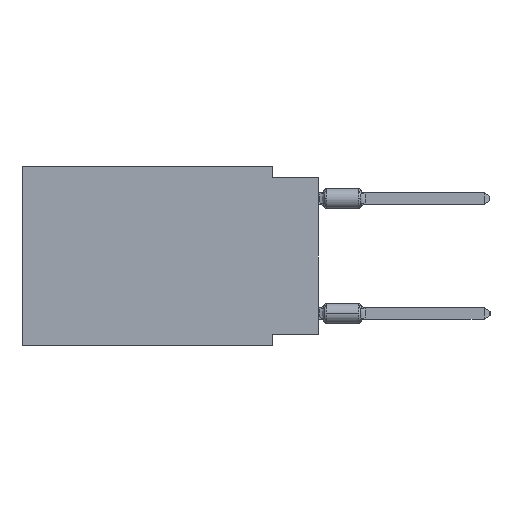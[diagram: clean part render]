
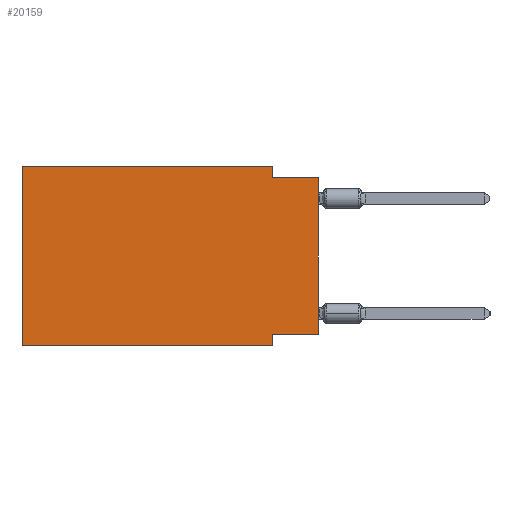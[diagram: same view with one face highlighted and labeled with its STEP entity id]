
A CAD part, left-side view. The second image highlights one B-rep face of the part: STEP entity #20159.
In plain terms, the highlighted planar face has unit normal (-1, 0, 0).
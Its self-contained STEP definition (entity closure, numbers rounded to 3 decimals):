
#829 = DIRECTION ( 'NONE',  ( 0., 0., -1. ) ) ;
#1576 = VERTEX_POINT ( 'NONE', #36113 ) ;
#1631 = ORIENTED_EDGE ( 'NONE', *, *, #31599, .T. ) ;
#2872 = VECTOR ( 'NONE', #36932, 1000. ) ;
#3342 = CARTESIAN_POINT ( 'NONE',  ( 0., 16.383, 0. ) ) ;
#4728 = CARTESIAN_POINT ( 'NONE',  ( 0., 0., -9.271 ) ) ;
#4975 = PLANE ( 'NONE',  #40222 ) ;
#6924 = VERTEX_POINT ( 'NONE', #50520 ) ;
#7307 = VERTEX_POINT ( 'NONE', #45856 ) ;
#8374 = VERTEX_POINT ( 'NONE', #40048 ) ;
#9286 = EDGE_LOOP ( 'NONE', ( #39511, #28582, #34691, #48635, #46377, #1631, #33042, #9824 ) ) ;
#9824 = ORIENTED_EDGE ( 'NONE', *, *, #44631, .F. ) ;
#10026 = CARTESIAN_POINT ( 'NONE',  ( 0., 16.383, 0. ) ) ;
#10186 = DIRECTION ( 'NONE',  ( 0., 0., -1. ) ) ;
#11229 = LINE ( 'NONE', #38233, #13995 ) ;
#12120 = VERTEX_POINT ( 'NONE', #58046 ) ;
#13102 = EDGE_CURVE ( 'NONE', #1576, #8374, #18227, .T. ) ;
#13995 = VECTOR ( 'NONE', #829, 1000. ) ;
#16010 = VECTOR ( 'NONE', #32621, 1000. ) ;
#18227 = LINE ( 'NONE', #41234, #2872 ) ;
#18235 = LINE ( 'NONE', #4728, #16010 ) ;
#19677 = FACE_OUTER_BOUND ( 'NONE', #9286, .T. ) ;
#19977 = EDGE_CURVE ( 'NONE', #7307, #20957, #27353, .T. ) ;
#20159 = ADVANCED_FACE ( 'NONE', ( #19677 ), #4975, .F. ) ;
#20957 = VERTEX_POINT ( 'NONE', #35305 ) ;
#23691 = VERTEX_POINT ( 'NONE', #58237 ) ;
#27317 = EDGE_CURVE ( 'NONE', #6924, #37958, #49645, .T. ) ;
#27353 = LINE ( 'NONE', #31956, #49989 ) ;
#28576 = DIRECTION ( 'NONE',  ( 1., 0., 0. ) ) ;
#28582 = ORIENTED_EDGE ( 'NONE', *, *, #40067, .F. ) ;
#28759 = CARTESIAN_POINT ( 'NONE',  ( 0., 2.54, 0. ) ) ;
#29307 = LINE ( 'NONE', #10026, #42438 ) ;
#31194 = CARTESIAN_POINT ( 'NONE',  ( 0., 16.383, -9.906 ) ) ;
#31599 = EDGE_CURVE ( 'NONE', #23691, #8374, #45617, .T. ) ;
#31956 = CARTESIAN_POINT ( 'NONE',  ( 0., 0., 0. ) ) ;
#31960 = VECTOR ( 'NONE', #39540, 1000. ) ;
#32621 = DIRECTION ( 'NONE',  ( 0., 1., 0. ) ) ;
#33042 = ORIENTED_EDGE ( 'NONE', *, *, #13102, .F. ) ;
#33664 = EDGE_CURVE ( 'NONE', #23691, #6924, #29307, .T. ) ;
#34691 = ORIENTED_EDGE ( 'NONE', *, *, #34711, .F. ) ;
#34711 = EDGE_CURVE ( 'NONE', #37958, #12120, #11229, .T. ) ;
#35305 = CARTESIAN_POINT ( 'NONE',  ( 0., 0., -0.635 ) ) ;
#36113 = CARTESIAN_POINT ( 'NONE',  ( 0., 2.54, -9.271 ) ) ;
#36932 = DIRECTION ( 'NONE',  ( 0., 0., -1. ) ) ;
#37958 = VERTEX_POINT ( 'NONE', #28759 ) ;
#38233 = CARTESIAN_POINT ( 'NONE',  ( 0., 2.54, 0. ) ) ;
#39511 = ORIENTED_EDGE ( 'NONE', *, *, #19977, .T. ) ;
#39540 = DIRECTION ( 'NONE',  ( 0., -1., 0. ) ) ;
#40048 = CARTESIAN_POINT ( 'NONE',  ( 0., 2.54, -9.906 ) ) ;
#40067 = EDGE_CURVE ( 'NONE', #12120, #20957, #42725, .T. ) ;
#40222 = AXIS2_PLACEMENT_3D ( 'NONE', #56488, #28576, #10186 ) ;
#41234 = CARTESIAN_POINT ( 'NONE',  ( 0., 2.54, -9.906 ) ) ;
#41776 = DIRECTION ( 'NONE',  ( 0., 0., 1. ) ) ;
#42438 = VECTOR ( 'NONE', #52906, 1000. ) ;
#42725 = LINE ( 'NONE', #60521, #44769 ) ;
#44631 = EDGE_CURVE ( 'NONE', #7307, #1576, #18235, .T. ) ;
#44769 = VECTOR ( 'NONE', #50722, 1000. ) ;
#45197 = VECTOR ( 'NONE', #49609, 1000. ) ;
#45617 = LINE ( 'NONE', #31194, #45197 ) ;
#45856 = CARTESIAN_POINT ( 'NONE',  ( 0., 0., -9.271 ) ) ;
#46377 = ORIENTED_EDGE ( 'NONE', *, *, #33664, .F. ) ;
#48635 = ORIENTED_EDGE ( 'NONE', *, *, #27317, .F. ) ;
#49609 = DIRECTION ( 'NONE',  ( 0., -1., 0. ) ) ;
#49645 = LINE ( 'NONE', #3342, #31960 ) ;
#49989 = VECTOR ( 'NONE', #41776, 1000. ) ;
#50520 = CARTESIAN_POINT ( 'NONE',  ( 0., 16.383, 0. ) ) ;
#50722 = DIRECTION ( 'NONE',  ( 0., -1., 0. ) ) ;
#52906 = DIRECTION ( 'NONE',  ( 0., 0., 1. ) ) ;
#56488 = CARTESIAN_POINT ( 'NONE',  ( 0., 16.383, 0. ) ) ;
#58046 = CARTESIAN_POINT ( 'NONE',  ( 0., 2.54, -0.635 ) ) ;
#58237 = CARTESIAN_POINT ( 'NONE',  ( 0., 16.383, -9.906 ) ) ;
#60521 = CARTESIAN_POINT ( 'NONE',  ( 0., 0., -0.635 ) ) ;
